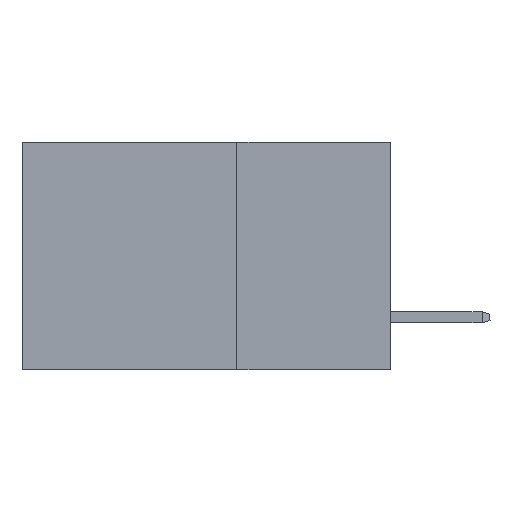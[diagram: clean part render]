
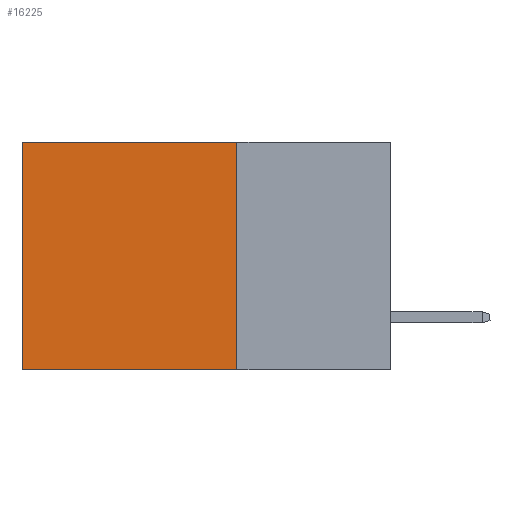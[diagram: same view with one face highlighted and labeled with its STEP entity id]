
A CAD part, left-side view. The second image highlights one B-rep face of the part: STEP entity #16225.
In plain terms, the highlighted planar face has unit normal (-1, 0, 0).
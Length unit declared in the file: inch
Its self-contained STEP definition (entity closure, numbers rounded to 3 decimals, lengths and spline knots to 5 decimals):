
#175 = CARTESIAN_POINT ( 'NONE',  ( 0.2875, 0.6, 0. ) ) ;
#257 = DIRECTION ( 'NONE',  ( 0., 0., -1. ) ) ;
#523 = ORIENTED_EDGE ( 'NONE', *, *, #1815, .T. ) ;
#581 = VECTOR ( 'NONE', #257, 39.37008 ) ;
#1189 = CARTESIAN_POINT ( 'NONE',  ( 0.2875, 0.6, -0.37 ) ) ;
#1787 = ORIENTED_EDGE ( 'NONE', *, *, #4960, .F. ) ;
#1815 = EDGE_CURVE ( 'NONE', #1872, #16485, #14554, .T. ) ;
#1872 = VERTEX_POINT ( 'NONE', #3323 ) ;
#2182 = CARTESIAN_POINT ( 'NONE',  ( 0.2875, 0.6, 0. ) ) ;
#2236 = EDGE_LOOP ( 'NONE', ( #12122, #13043, #1787, #523 ) ) ;
#2398 = VERTEX_POINT ( 'NONE', #12253 ) ;
#3079 = CARTESIAN_POINT ( 'NONE',  ( 0.2875, 0.25, 0. ) ) ;
#3323 = CARTESIAN_POINT ( 'NONE',  ( 0.2875, 0.25, 0. ) ) ;
#4518 = CARTESIAN_POINT ( 'NONE',  ( 0.2875, 0.25, 0. ) ) ;
#4960 = EDGE_CURVE ( 'NONE', #1872, #2398, #16078, .T. ) ;
#5143 = DIRECTION ( 'NONE',  ( 0., 0., -1. ) ) ;
#5230 = CARTESIAN_POINT ( 'NONE',  ( 0.2875, 0.25, 0. ) ) ;
#6590 = EDGE_CURVE ( 'NONE', #2398, #11211, #7049, .T. ) ;
#6888 = DIRECTION ( 'NONE',  ( 0., 1., 0. ) ) ;
#7049 = LINE ( 'NONE', #11015, #8197 ) ;
#8197 = VECTOR ( 'NONE', #6888, 39.37008 ) ;
#9671 = DIRECTION ( 'NONE',  ( 0., 0., -1. ) ) ;
#10384 = PLANE ( 'NONE',  #15374 ) ;
#10671 = VECTOR ( 'NONE', #9671, 39.37008 ) ;
#10842 = DIRECTION ( 'NONE',  ( 0., 1., 0. ) ) ;
#11015 = CARTESIAN_POINT ( 'NONE',  ( 0.2875, 0.25, -0.37 ) ) ;
#11211 = VERTEX_POINT ( 'NONE', #1189 ) ;
#11983 = FACE_OUTER_BOUND ( 'NONE', #2236, .T. ) ;
#12122 = ORIENTED_EDGE ( 'NONE', *, *, #16585, .T. ) ;
#12253 = CARTESIAN_POINT ( 'NONE',  ( 0.2875, 0.25, -0.37 ) ) ;
#13043 = ORIENTED_EDGE ( 'NONE', *, *, #6590, .F. ) ;
#14554 = LINE ( 'NONE', #3079, #15025 ) ;
#15025 = VECTOR ( 'NONE', #10842, 39.37008 ) ;
#15374 = AXIS2_PLACEMENT_3D ( 'NONE', #5230, #15688, #5143 ) ;
#15670 = LINE ( 'NONE', #175, #581 ) ;
#15688 = DIRECTION ( 'NONE',  ( 1., 0., 0. ) ) ;
#16078 = LINE ( 'NONE', #4518, #10671 ) ;
#16225 = ADVANCED_FACE ( 'NONE', ( #11983 ), #10384, .F. ) ;
#16485 = VERTEX_POINT ( 'NONE', #2182 ) ;
#16585 = EDGE_CURVE ( 'NONE', #16485, #11211, #15670, .T. ) ;
